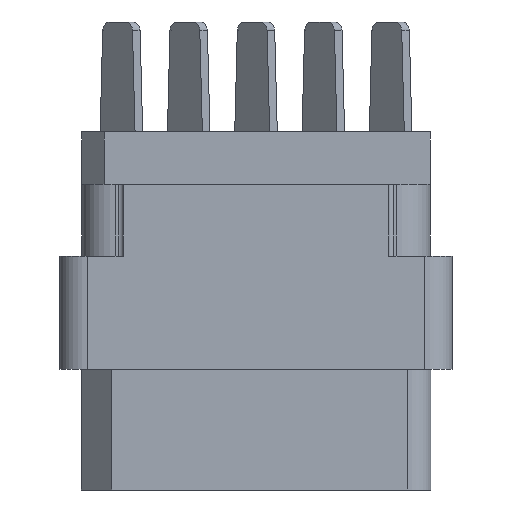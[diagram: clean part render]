
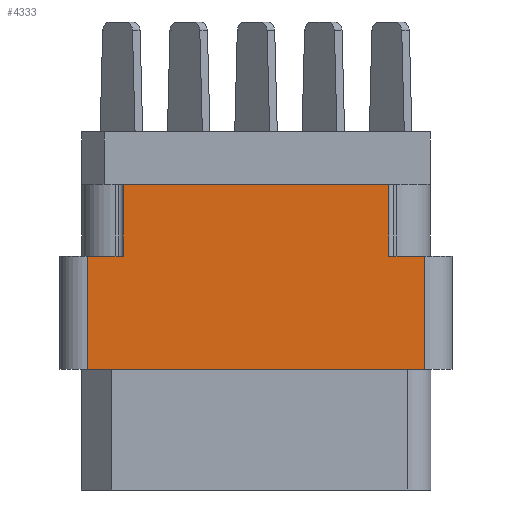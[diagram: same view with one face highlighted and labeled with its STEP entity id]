
A CAD part, left-side view. The second image highlights one B-rep face of the part: STEP entity #4333.
In plain terms, the highlighted planar face has unit normal (-1, 0, 0).
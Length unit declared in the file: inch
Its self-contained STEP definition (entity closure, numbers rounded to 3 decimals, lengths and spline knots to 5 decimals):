
#137 = LINE ( 'NONE', #10112, #625 ) ;
#305 = CARTESIAN_POINT ( 'NONE',  ( -1., -0.376, -0.798 ) ) ;
#625 = VECTOR ( 'NONE', #7669, 39.37008 ) ;
#1206 = ORIENTED_EDGE ( 'NONE', *, *, #12067, .F. ) ;
#1365 = VECTOR ( 'NONE', #12790, 39.37008 ) ;
#1383 = PLANE ( 'NONE',  #10197 ) ;
#1668 = DIRECTION ( 'NONE',  ( 0., 0., 1. ) ) ;
#1895 = VECTOR ( 'NONE', #18254, 39.37008 ) ;
#2012 = CARTESIAN_POINT ( 'NONE',  ( -1., 0.376, -0.277 ) ) ;
#2538 = EDGE_CURVE ( 'NONE', #6560, #5199, #31384, .T. ) ;
#2702 = ORIENTED_EDGE ( 'NONE', *, *, #11564, .F. ) ;
#2925 = DIRECTION ( 'NONE',  ( 0., 1., 0. ) ) ;
#3223 = VERTEX_POINT ( 'NONE', #14869 ) ;
#4333 = ADVANCED_FACE ( 'NONE', ( #5962 ), #1383, .T. ) ;
#5029 = EDGE_CURVE ( 'NONE', #26872, #3223, #22982, .T. ) ;
#5096 = EDGE_CURVE ( 'NONE', #5199, #7265, #137, .T. ) ;
#5107 = EDGE_CURVE ( 'NONE', #26872, #21924, #15315, .T. ) ;
#5199 = VERTEX_POINT ( 'NONE', #18886 ) ;
#5962 = FACE_OUTER_BOUND ( 'NONE', #24813, .T. ) ;
#6289 = DIRECTION ( 'NONE',  ( 0., 0., 1. ) ) ;
#6560 = VERTEX_POINT ( 'NONE', #21387 ) ;
#7265 = VERTEX_POINT ( 'NONE', #13950 ) ;
#7273 = CARTESIAN_POINT ( 'NONE',  ( -1., -0.296, -0.277 ) ) ;
#7547 = VECTOR ( 'NONE', #1668, 39.37008 ) ;
#7669 = DIRECTION ( 'NONE',  ( 0., -1., 0. ) ) ;
#7927 = VECTOR ( 'NONE', #2925, 39.37008 ) ;
#8647 = LINE ( 'NONE', #31164, #26197 ) ;
#9552 = CARTESIAN_POINT ( 'NONE',  ( -1., 0.376, -0.529 ) ) ;
#9767 = CARTESIAN_POINT ( 'NONE',  ( -1., -0.296, -0.277 ) ) ;
#10065 = EDGE_CURVE ( 'NONE', #12455, #7265, #32291, .T. ) ;
#10112 = CARTESIAN_POINT ( 'NONE',  ( -1., 0.438, -0.117 ) ) ;
#10197 = AXIS2_PLACEMENT_3D ( 'NONE', #18845, #30924, #6289 ) ;
#10558 = ORIENTED_EDGE ( 'NONE', *, *, #5107, .F. ) ;
#10804 = CARTESIAN_POINT ( 'NONE',  ( -1., 0.438, -0.277 ) ) ;
#11564 = EDGE_CURVE ( 'NONE', #26240, #6560, #15207, .T. ) ;
#12067 = EDGE_CURVE ( 'NONE', #21924, #26240, #8647, .T. ) ;
#12455 = VERTEX_POINT ( 'NONE', #18991 ) ;
#12790 = DIRECTION ( 'NONE',  ( 0., -1., 0. ) ) ;
#13228 = DIRECTION ( 'NONE',  ( 0., -1., 0. ) ) ;
#13950 = CARTESIAN_POINT ( 'NONE',  ( -1., -0.296, -0.117 ) ) ;
#14869 = CARTESIAN_POINT ( 'NONE',  ( -1., -0.376, -0.277 ) ) ;
#15136 = ORIENTED_EDGE ( 'NONE', *, *, #10065, .T. ) ;
#15207 = LINE ( 'NONE', #10804, #23113 ) ;
#15315 = LINE ( 'NONE', #25278, #7927 ) ;
#15459 = ORIENTED_EDGE ( 'NONE', *, *, #2538, .F. ) ;
#16326 = VECTOR ( 'NONE', #29671, 39.37008 ) ;
#17038 = ORIENTED_EDGE ( 'NONE', *, *, #5096, .F. ) ;
#17220 = ORIENTED_EDGE ( 'NONE', *, *, #5029, .T. ) ;
#18254 = DIRECTION ( 'NONE',  ( 0., 0., 1. ) ) ;
#18313 = ORIENTED_EDGE ( 'NONE', *, *, #20825, .F. ) ;
#18845 = CARTESIAN_POINT ( 'NONE',  ( -1., -0.376, -0.798 ) ) ;
#18886 = CARTESIAN_POINT ( 'NONE',  ( -1., 0.296, -0.117 ) ) ;
#18991 = CARTESIAN_POINT ( 'NONE',  ( -1., -0.296, -0.277 ) ) ;
#20348 = CARTESIAN_POINT ( 'NONE',  ( -1., -0.376, -0.529 ) ) ;
#20825 = EDGE_CURVE ( 'NONE', #12455, #3223, #22274, .T. ) ;
#21387 = CARTESIAN_POINT ( 'NONE',  ( -1., 0.296, -0.277 ) ) ;
#21924 = VERTEX_POINT ( 'NONE', #9552 ) ;
#22274 = LINE ( 'NONE', #7273, #1365 ) ;
#22982 = LINE ( 'NONE', #305, #1895 ) ;
#23113 = VECTOR ( 'NONE', #13228, 39.37008 ) ;
#24813 = EDGE_LOOP ( 'NONE', ( #1206, #10558, #17220, #18313, #15136, #17038, #15459, #2702 ) ) ;
#25278 = CARTESIAN_POINT ( 'NONE',  ( -1., -0.376, -0.529 ) ) ;
#26197 = VECTOR ( 'NONE', #28387, 39.37008 ) ;
#26240 = VERTEX_POINT ( 'NONE', #2012 ) ;
#26872 = VERTEX_POINT ( 'NONE', #20348 ) ;
#28387 = DIRECTION ( 'NONE',  ( 0., 0., 1. ) ) ;
#29671 = DIRECTION ( 'NONE',  ( 0., 0., 1. ) ) ;
#30924 = DIRECTION ( 'NONE',  ( -1., 0., 0. ) ) ;
#31164 = CARTESIAN_POINT ( 'NONE',  ( -1., 0.376, -0.798 ) ) ;
#31384 = LINE ( 'NONE', #31552, #7547 ) ;
#31552 = CARTESIAN_POINT ( 'NONE',  ( -1., 0.296, -0.277 ) ) ;
#32291 = LINE ( 'NONE', #9767, #16326 ) ;
